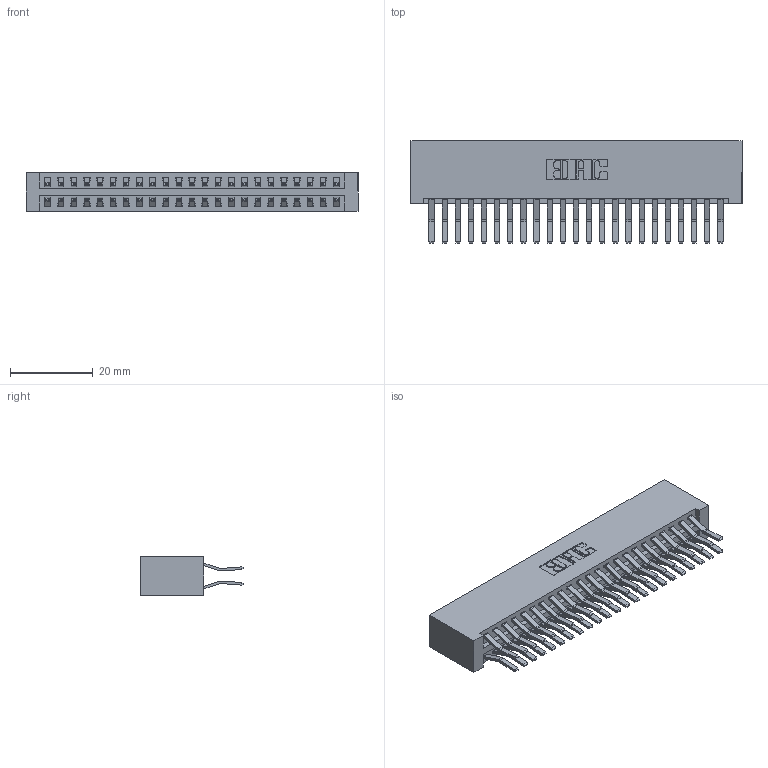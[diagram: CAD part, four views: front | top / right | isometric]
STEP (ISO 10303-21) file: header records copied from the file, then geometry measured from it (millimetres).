
FILE_DESCRIPTION (( 'STEP AP203' ), '1' );
FILE_NAME ('396-046-560-201.STEP', '2018-09-07T09:56:56', ( '' ), ( '' ), 'SwSTEP 2.0', 'SolidWorks 2016', '' );
FILE_SCHEMA (( 'CONFIG_CONTROL_DESIGN' ));
Length unit declared in the file: inch
Products named in the file (3): 346 Part_No Mounting Lugs; 345-292-001_560 Tail; 396-046-560-201
Assembly tree (47 placements, depth 2):
  396-046-560-201
    346 Part_No Mounting Lugs
    345-292-001_560 Tail  x46
Bounding box: 80.26 x 24.78 x 9.4 mm (x, y, z)
Volume: 8554 mm3; surface area: 12427 mm2
Topology: 47 solids, 47 shells, 2598 faces, 7711 edges, 5078 vertices
Faces by surface type: plane 1682, cylinder 916
Entity records: 17379 total; most frequent: CARTESIAN_POINT 2888, ORIENTED_EDGE 2822, DIRECTION 2595, EDGE_CURVE 1411, VECTOR 1191, LINE 1191, VERTEX_POINT 938, AXIS2_PLACEMENT_3D 702
